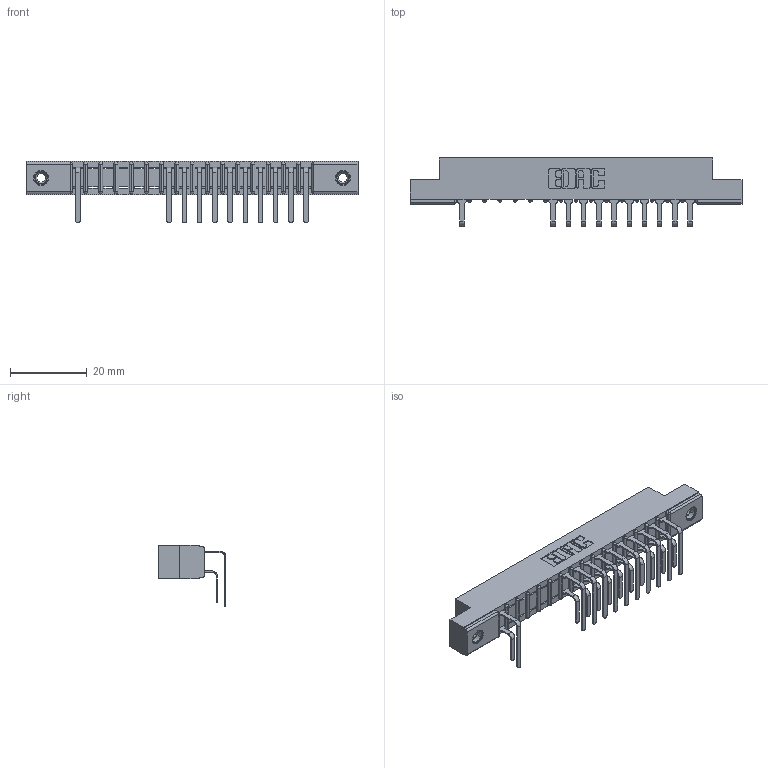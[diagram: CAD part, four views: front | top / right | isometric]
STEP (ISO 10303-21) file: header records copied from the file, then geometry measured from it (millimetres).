
FILE_DESCRIPTION (( 'STEP AP203' ), '1' );
FILE_NAME ('307-016-559-108.STEP', '2018-08-03T03:10:20', ( '' ), ( '' ), 'SwSTEP 2.0', 'SolidWorks 2016', '' );
FILE_SCHEMA (( 'CONFIG_CONTROL_DESIGN' ));
Length unit declared in the file: inch
Products named in the file (5): 307-290-001_559 - 2 (Single); 345-250-001_345-250-003-102; 307-016-559-108; 307 Part_.156 Dia Mounting Holes; 307-290-001_558 559 - 1 (Single)
Assembly tree (25 placements, depth 2):
  307-016-559-108
    307 Part_.156 Dia Mounting Holes
    307-290-001_558 559 - 1 (Single)  x11
    307-290-001_559 - 2 (Single)  x11
    345-250-001_345-250-003-102  x2
Bounding box: 86.41 x 17.69 x 16.08 mm (x, y, z)
Volume: 5614.4 mm3; surface area: 9409.6 mm2
Topology: 25 solids, 25 shells, 1395 faces, 3903 edges, 2518 vertices
Faces by surface type: plane 888, cylinder 457, sphere 34, cone 12, torus 4
Entity records: 19746 total; most frequent: CARTESIAN_POINT 3267, ORIENTED_EDGE 3238, DIRECTION 3209, EDGE_CURVE 1619, VECTOR 1229, LINE 1229, VERTEX_POINT 1048, AXIS2_PLACEMENT_3D 990
